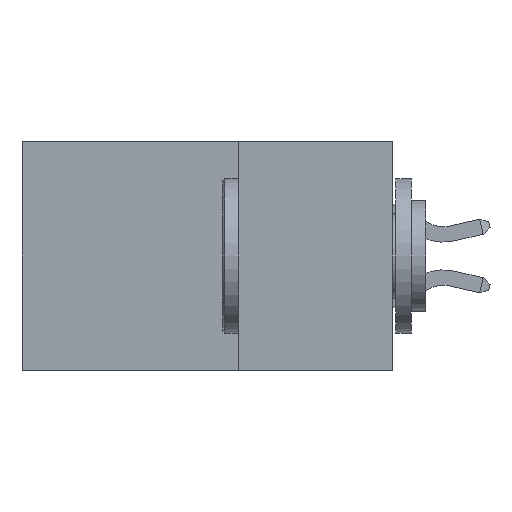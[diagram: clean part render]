
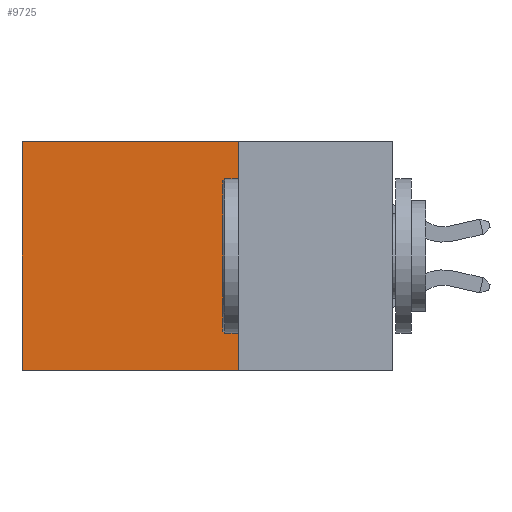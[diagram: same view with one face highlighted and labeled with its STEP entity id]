
A CAD part, left-side view. The second image highlights one B-rep face of the part: STEP entity #9725.
In plain terms, the highlighted planar face has unit normal (-1, 0, 0).
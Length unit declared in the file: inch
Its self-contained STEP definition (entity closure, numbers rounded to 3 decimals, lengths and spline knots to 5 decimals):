
#308 = DIRECTION ( 'NONE',  ( 0., 0., -1. ) ) ;
#455 = VECTOR ( 'NONE', #3155, 39.37008 ) ;
#531 = ORIENTED_EDGE ( 'NONE', *, *, #4463, .F. ) ;
#865 = LINE ( 'NONE', #2940, #4527 ) ;
#1562 = ORIENTED_EDGE ( 'NONE', *, *, #9403, .T. ) ;
#1763 = PLANE ( 'NONE',  #9679 ) ;
#2086 = DIRECTION ( 'NONE',  ( 0., 0., -1. ) ) ;
#2235 = LINE ( 'NONE', #9235, #3904 ) ;
#2566 = DIRECTION ( 'NONE',  ( 1., 0., 0. ) ) ;
#2598 = VERTEX_POINT ( 'NONE', #7996 ) ;
#2940 = CARTESIAN_POINT ( 'NONE',  ( 0.2875, 0.25, 0. ) ) ;
#3155 = DIRECTION ( 'NONE',  ( 0., 1., 0. ) ) ;
#3596 = FACE_OUTER_BOUND ( 'NONE', #6978, .T. ) ;
#3611 = CARTESIAN_POINT ( 'NONE',  ( 0.2875, 0.25, -0.37 ) ) ;
#3707 = CARTESIAN_POINT ( 'NONE',  ( 0.2875, 0.6, -0.37 ) ) ;
#3874 = VERTEX_POINT ( 'NONE', #3707 ) ;
#3904 = VECTOR ( 'NONE', #6968, 39.37008 ) ;
#3916 = ORIENTED_EDGE ( 'NONE', *, *, #9885, .T. ) ;
#4463 = EDGE_CURVE ( 'NONE', #6750, #3874, #2235, .T. ) ;
#4527 = VECTOR ( 'NONE', #2086, 39.37008 ) ;
#4529 = EDGE_CURVE ( 'NONE', #2598, #6750, #865, .T. ) ;
#4739 = LINE ( 'NONE', #6480, #455 ) ;
#5021 = CARTESIAN_POINT ( 'NONE',  ( 0.2875, 0.25, 0. ) ) ;
#5489 = ORIENTED_EDGE ( 'NONE', *, *, #4529, .F. ) ;
#5647 = CARTESIAN_POINT ( 'NONE',  ( 0.2875, 0.6, 0. ) ) ;
#6202 = VERTEX_POINT ( 'NONE', #8520 ) ;
#6480 = CARTESIAN_POINT ( 'NONE',  ( 0.2875, 0.25, 0. ) ) ;
#6505 = DIRECTION ( 'NONE',  ( 0., 0., -1. ) ) ;
#6750 = VERTEX_POINT ( 'NONE', #3611 ) ;
#6968 = DIRECTION ( 'NONE',  ( 0., 1., 0. ) ) ;
#6978 = EDGE_LOOP ( 'NONE', ( #1562, #531, #5489, #3916 ) ) ;
#7996 = CARTESIAN_POINT ( 'NONE',  ( 0.2875, 0.25, 0. ) ) ;
#8520 = CARTESIAN_POINT ( 'NONE',  ( 0.2875, 0.6, 0. ) ) ;
#8726 = LINE ( 'NONE', #5647, #10103 ) ;
#9235 = CARTESIAN_POINT ( 'NONE',  ( 0.2875, 0.25, -0.37 ) ) ;
#9403 = EDGE_CURVE ( 'NONE', #6202, #3874, #8726, .T. ) ;
#9679 = AXIS2_PLACEMENT_3D ( 'NONE', #5021, #2566, #308 ) ;
#9725 = ADVANCED_FACE ( 'NONE', ( #3596 ), #1763, .F. ) ;
#9885 = EDGE_CURVE ( 'NONE', #2598, #6202, #4739, .T. ) ;
#10103 = VECTOR ( 'NONE', #6505, 39.37008 ) ;
